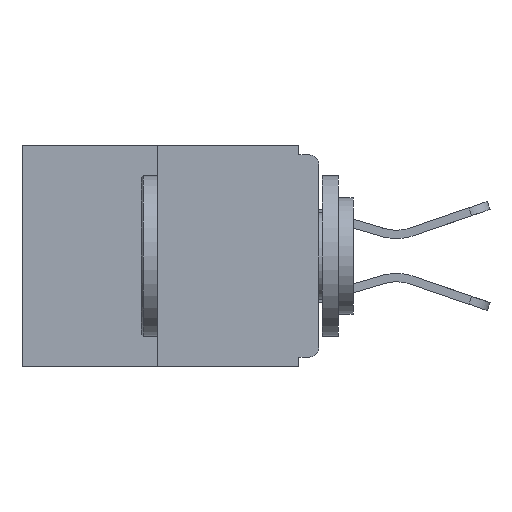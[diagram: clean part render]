
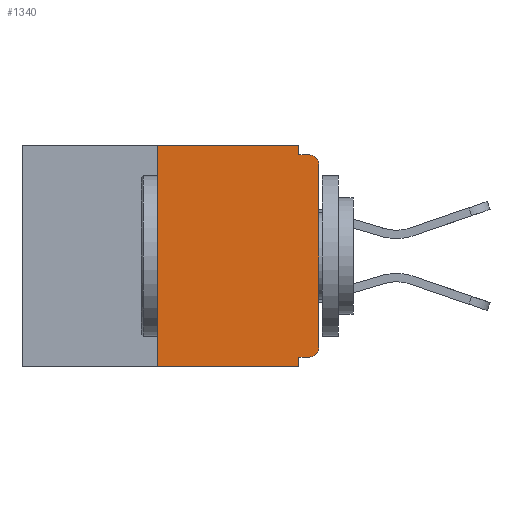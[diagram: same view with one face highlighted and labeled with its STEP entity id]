
A CAD part, left-side view. The second image highlights one B-rep face of the part: STEP entity #1340.
In plain terms, the highlighted planar face has unit normal (-1, 0, 0).
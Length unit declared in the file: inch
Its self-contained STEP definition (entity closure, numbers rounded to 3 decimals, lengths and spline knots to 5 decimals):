
#717 = DIRECTION ( 'NONE',  ( -1., 0., 0. ) ) ;
#751 = CARTESIAN_POINT ( 'NONE',  ( 0., 0., -0.328 ) ) ;
#1340 = ADVANCED_FACE ( 'NONE', ( #23656 ), #15000, .F. ) ;
#1464 = DIRECTION ( 'NONE',  ( 0., -1., 0. ) ) ;
#1922 = VERTEX_POINT ( 'NONE', #11086 ) ;
#2012 = EDGE_CURVE ( 'NONE', #25210, #2721, #17926, .T. ) ;
#2214 = CARTESIAN_POINT ( 'NONE',  ( 0., 0.015, -0.015 ) ) ;
#2529 = ORIENTED_EDGE ( 'NONE', *, *, #4907, .T. ) ;
#2721 = VERTEX_POINT ( 'NONE', #2214 ) ;
#3045 = CARTESIAN_POINT ( 'NONE',  ( 0., 0.015, -0.328 ) ) ;
#3332 = EDGE_CURVE ( 'NONE', #14176, #5744, #13134, .T. ) ;
#3642 = AXIS2_PLACEMENT_3D ( 'NONE', #17172, #21464, #12930 ) ;
#3699 = CARTESIAN_POINT ( 'NONE',  ( 0., 0.46, 0. ) ) ;
#4907 = EDGE_CURVE ( 'NONE', #23234, #5744, #14800, .T. ) ;
#5139 = AXIS2_PLACEMENT_3D ( 'NONE', #26554, #717, #20100 ) ;
#5254 = CARTESIAN_POINT ( 'NONE',  ( 0., 0.25, 0. ) ) ;
#5587 = LINE ( 'NONE', #23031, #19421 ) ;
#5744 = VERTEX_POINT ( 'NONE', #7507 ) ;
#5954 = LINE ( 'NONE', #5254, #16444 ) ;
#6148 = EDGE_CURVE ( 'NONE', #10293, #16356, #27611, .T. ) ;
#7247 = CARTESIAN_POINT ( 'NONE',  ( 0., 0., -0.015 ) ) ;
#7507 = CARTESIAN_POINT ( 'NONE',  ( 0., 0.031, -0.343 ) ) ;
#7698 = VECTOR ( 'NONE', #1464, 39.37008 ) ;
#7825 = CARTESIAN_POINT ( 'NONE',  ( 0., 0., -0.03 ) ) ;
#7903 = CARTESIAN_POINT ( 'NONE',  ( 0., 0.015, -0.313 ) ) ;
#8106 = VECTOR ( 'NONE', #9048, 39.37008 ) ;
#8148 = CARTESIAN_POINT ( 'NONE',  ( 0., 0.031, -0.328 ) ) ;
#8803 = LINE ( 'NONE', #751, #8106 ) ;
#9046 = ORIENTED_EDGE ( 'NONE', *, *, #17567, .F. ) ;
#9048 = DIRECTION ( 'NONE',  ( 0., 1., 0. ) ) ;
#9779 = DIRECTION ( 'NONE',  ( 0., -1., 0. ) ) ;
#10293 = VERTEX_POINT ( 'NONE', #3045 ) ;
#10366 = EDGE_CURVE ( 'NONE', #13334, #2721, #16996, .T. ) ;
#10410 = ORIENTED_EDGE ( 'NONE', *, *, #3332, .F. ) ;
#11086 = CARTESIAN_POINT ( 'NONE',  ( 0., 0.25, 0. ) ) ;
#11113 = VERTEX_POINT ( 'NONE', #11629 ) ;
#11273 = VECTOR ( 'NONE', #11891, 39.37008 ) ;
#11629 = CARTESIAN_POINT ( 'NONE',  ( 0., 0.031, 0. ) ) ;
#11673 = LINE ( 'NONE', #3699, #12347 ) ;
#11891 = DIRECTION ( 'NONE',  ( 0., -1., 0. ) ) ;
#11959 = EDGE_CURVE ( 'NONE', #23234, #1922, #5954, .T. ) ;
#12347 = VECTOR ( 'NONE', #9779, 39.37008 ) ;
#12930 = DIRECTION ( 'NONE',  ( 0., 0., -1. ) ) ;
#13134 = LINE ( 'NONE', #21028, #22521 ) ;
#13334 = VERTEX_POINT ( 'NONE', #15824 ) ;
#13687 = CARTESIAN_POINT ( 'NONE',  ( 0., 0., -0.313 ) ) ;
#14176 = VERTEX_POINT ( 'NONE', #8148 ) ;
#14430 = DIRECTION ( 'NONE',  ( 0., 0., -1. ) ) ;
#14706 = EDGE_CURVE ( 'NONE', #11113, #13334, #16610, .T. ) ;
#14800 = LINE ( 'NONE', #27305, #7698 ) ;
#15000 = PLANE ( 'NONE',  #3642 ) ;
#15090 = ORIENTED_EDGE ( 'NONE', *, *, #14706, .F. ) ;
#15824 = CARTESIAN_POINT ( 'NONE',  ( 0., 0.031, -0.015 ) ) ;
#16112 = DIRECTION ( 'NONE',  ( 0., 0., 1. ) ) ;
#16356 = VERTEX_POINT ( 'NONE', #13687 ) ;
#16444 = VECTOR ( 'NONE', #16112, 39.37008 ) ;
#16610 = LINE ( 'NONE', #18666, #19306 ) ;
#16996 = LINE ( 'NONE', #7247, #11273 ) ;
#17172 = CARTESIAN_POINT ( 'NONE',  ( 0., 0.46, 0. ) ) ;
#17567 = EDGE_CURVE ( 'NONE', #10293, #14176, #8803, .T. ) ;
#17926 = CIRCLE ( 'NONE', #5139, 0.015 ) ;
#18666 = CARTESIAN_POINT ( 'NONE',  ( 0., 0.031, 0. ) ) ;
#19306 = VECTOR ( 'NONE', #20730, 39.37008 ) ;
#19421 = VECTOR ( 'NONE', #20901, 39.37008 ) ;
#20100 = DIRECTION ( 'NONE',  ( 0., 0., -1. ) ) ;
#20730 = DIRECTION ( 'NONE',  ( 0., 0., -1. ) ) ;
#20901 = DIRECTION ( 'NONE',  ( 0., 0., 1. ) ) ;
#20926 = ORIENTED_EDGE ( 'NONE', *, *, #25659, .F. ) ;
#21028 = CARTESIAN_POINT ( 'NONE',  ( 0., 0.031, -0.343 ) ) ;
#21464 = DIRECTION ( 'NONE',  ( 1., 0., 0. ) ) ;
#21625 = EDGE_LOOP ( 'NONE', ( #20926, #23613, #2529, #10410, #9046, #21952, #24852, #21880, #25622, #15090 ) ) ;
#21880 = ORIENTED_EDGE ( 'NONE', *, *, #2012, .T. ) ;
#21952 = ORIENTED_EDGE ( 'NONE', *, *, #6148, .T. ) ;
#22110 = CARTESIAN_POINT ( 'NONE',  ( 0., 0.25, -0.343 ) ) ;
#22521 = VECTOR ( 'NONE', #25343, 39.37008 ) ;
#23031 = CARTESIAN_POINT ( 'NONE',  ( 0., 0., 0. ) ) ;
#23234 = VERTEX_POINT ( 'NONE', #22110 ) ;
#23613 = ORIENTED_EDGE ( 'NONE', *, *, #11959, .F. ) ;
#23656 = FACE_OUTER_BOUND ( 'NONE', #21625, .T. ) ;
#24024 = AXIS2_PLACEMENT_3D ( 'NONE', #7903, #25292, #14430 ) ;
#24852 = ORIENTED_EDGE ( 'NONE', *, *, #25265, .T. ) ;
#25210 = VERTEX_POINT ( 'NONE', #7825 ) ;
#25265 = EDGE_CURVE ( 'NONE', #16356, #25210, #5587, .T. ) ;
#25292 = DIRECTION ( 'NONE',  ( -1., 0., 0. ) ) ;
#25343 = DIRECTION ( 'NONE',  ( 0., 0., -1. ) ) ;
#25622 = ORIENTED_EDGE ( 'NONE', *, *, #10366, .F. ) ;
#25659 = EDGE_CURVE ( 'NONE', #1922, #11113, #11673, .T. ) ;
#26554 = CARTESIAN_POINT ( 'NONE',  ( 0., 0.015, -0.03 ) ) ;
#27305 = CARTESIAN_POINT ( 'NONE',  ( 0., 0.46, -0.343 ) ) ;
#27611 = CIRCLE ( 'NONE', #24024, 0.015 ) ;
